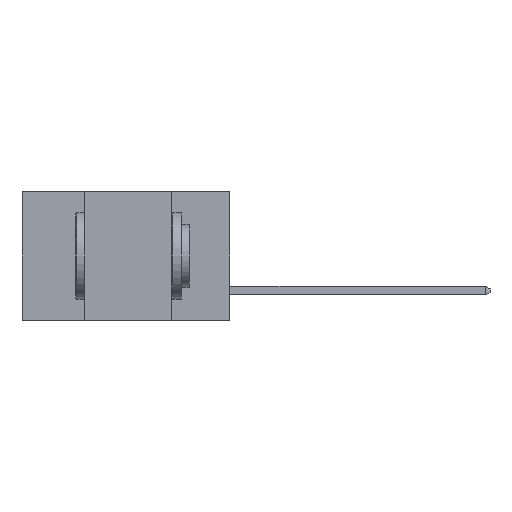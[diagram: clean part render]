
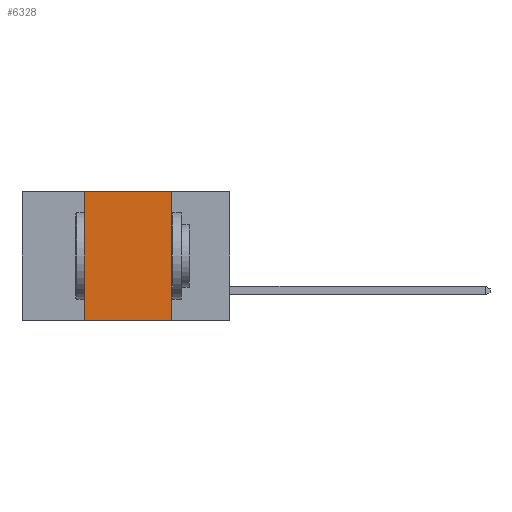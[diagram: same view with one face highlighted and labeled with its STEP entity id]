
A CAD part, left-side view. The second image highlights one B-rep face of the part: STEP entity #6328.
In plain terms, the highlighted planar face has unit normal (-1, 0, 0).
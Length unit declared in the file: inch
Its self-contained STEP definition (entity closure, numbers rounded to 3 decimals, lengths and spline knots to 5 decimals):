
#362 = ORIENTED_EDGE ( 'NONE', *, *, #1874, .F. ) ;
#490 = PLANE ( 'NONE',  #1875 ) ;
#655 = VERTEX_POINT ( 'NONE', #14392 ) ;
#930 = DIRECTION ( 'NONE',  ( 0., -1., 0. ) ) ;
#1302 = VECTOR ( 'NONE', #930, 39.37008 ) ;
#1493 = CARTESIAN_POINT ( 'NONE',  ( 0., 0.42, -0.37 ) ) ;
#1552 = DIRECTION ( 'NONE',  ( 0., 0., -1. ) ) ;
#1874 = EDGE_CURVE ( 'NONE', #4537, #655, #8820, .T. ) ;
#1875 = AXIS2_PLACEMENT_3D ( 'NONE', #3850, #12932, #1552 ) ;
#3752 = CARTESIAN_POINT ( 'NONE',  ( 0., 0.17, 0. ) ) ;
#3850 = CARTESIAN_POINT ( 'NONE',  ( 0., 0.6, 0. ) ) ;
#4005 = CARTESIAN_POINT ( 'NONE',  ( 0., 0.42, 0. ) ) ;
#4503 = LINE ( 'NONE', #13535, #11795 ) ;
#4537 = VERTEX_POINT ( 'NONE', #3752 ) ;
#4831 = LINE ( 'NONE', #1493, #9646 ) ;
#4894 = EDGE_LOOP ( 'NONE', ( #362, #6269, #4906, #10341 ) ) ;
#4906 = ORIENTED_EDGE ( 'NONE', *, *, #11346, .F. ) ;
#5776 = VECTOR ( 'NONE', #9315, 39.37008 ) ;
#6269 = ORIENTED_EDGE ( 'NONE', *, *, #10679, .F. ) ;
#6328 = ADVANCED_FACE ( 'NONE', ( #7610 ), #490, .F. ) ;
#6850 = LINE ( 'NONE', #14720, #1302 ) ;
#7242 = CARTESIAN_POINT ( 'NONE',  ( 0., 0.42, -0.37 ) ) ;
#7610 = FACE_OUTER_BOUND ( 'NONE', #4894, .T. ) ;
#7899 = DIRECTION ( 'NONE',  ( 0., -1., 0. ) ) ;
#7952 = VERTEX_POINT ( 'NONE', #4005 ) ;
#8820 = LINE ( 'NONE', #13826, #5776 ) ;
#9315 = DIRECTION ( 'NONE',  ( 0., 0., -1. ) ) ;
#9646 = VECTOR ( 'NONE', #11757, 39.37008 ) ;
#10279 = EDGE_CURVE ( 'NONE', #14534, #655, #6850, .T. ) ;
#10341 = ORIENTED_EDGE ( 'NONE', *, *, #10279, .T. ) ;
#10679 = EDGE_CURVE ( 'NONE', #7952, #4537, #4503, .T. ) ;
#11346 = EDGE_CURVE ( 'NONE', #14534, #7952, #4831, .T. ) ;
#11757 = DIRECTION ( 'NONE',  ( 0., 0., 1. ) ) ;
#11795 = VECTOR ( 'NONE', #7899, 39.37008 ) ;
#12932 = DIRECTION ( 'NONE',  ( 1., 0., 0. ) ) ;
#13535 = CARTESIAN_POINT ( 'NONE',  ( 0., 0.6, 0. ) ) ;
#13826 = CARTESIAN_POINT ( 'NONE',  ( 0., 0.17, -0.37 ) ) ;
#14392 = CARTESIAN_POINT ( 'NONE',  ( 0., 0.17, -0.37 ) ) ;
#14534 = VERTEX_POINT ( 'NONE', #7242 ) ;
#14720 = CARTESIAN_POINT ( 'NONE',  ( 0., 0.6, -0.37 ) ) ;
